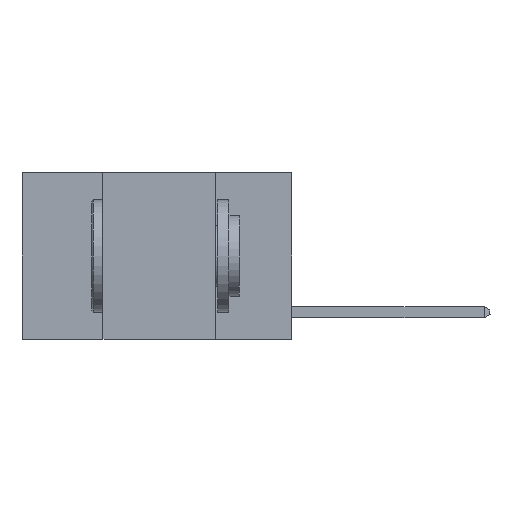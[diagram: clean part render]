
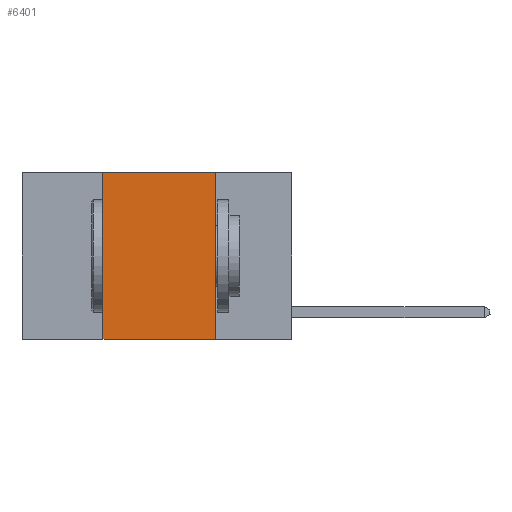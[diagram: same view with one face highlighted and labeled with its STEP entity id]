
A CAD part, left-side view. The second image highlights one B-rep face of the part: STEP entity #6401.
In plain terms, the highlighted planar face has unit normal (-1, 0, 0).
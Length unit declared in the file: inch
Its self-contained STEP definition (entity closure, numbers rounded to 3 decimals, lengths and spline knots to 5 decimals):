
#326 = CARTESIAN_POINT ( 'NONE',  ( 0., 0.42, 0. ) ) ;
#2627 = VECTOR ( 'NONE', #6405, 39.37008 ) ;
#2744 = CARTESIAN_POINT ( 'NONE',  ( 0., 0.17, -0.37 ) ) ;
#3440 = VERTEX_POINT ( 'NONE', #12475 ) ;
#3453 = VERTEX_POINT ( 'NONE', #2744 ) ;
#3882 = LINE ( 'NONE', #13676, #13071 ) ;
#4671 = ORIENTED_EDGE ( 'NONE', *, *, #11369, .T. ) ;
#5184 = CARTESIAN_POINT ( 'NONE',  ( 0., 0.6, 0. ) ) ;
#5519 = CARTESIAN_POINT ( 'NONE',  ( 0., 0.6, 0. ) ) ;
#5595 = EDGE_LOOP ( 'NONE', ( #15292, #9156, #9131, #4671 ) ) ;
#5746 = DIRECTION ( 'NONE',  ( 0., -1., 0. ) ) ;
#6401 = ADVANCED_FACE ( 'NONE', ( #8897 ), #11085, .F. ) ;
#6405 = DIRECTION ( 'NONE',  ( 0., 0., 1. ) ) ;
#6480 = LINE ( 'NONE', #12525, #2627 ) ;
#6493 = DIRECTION ( 'NONE',  ( 0., 0., -1. ) ) ;
#6754 = LINE ( 'NONE', #5519, #8022 ) ;
#7380 = CARTESIAN_POINT ( 'NONE',  ( 0., 0.17, 0. ) ) ;
#8022 = VECTOR ( 'NONE', #5746, 39.37008 ) ;
#8108 = EDGE_CURVE ( 'NONE', #14585, #9340, #6480, .T. ) ;
#8481 = DIRECTION ( 'NONE',  ( 0., 0., -1. ) ) ;
#8618 = DIRECTION ( 'NONE',  ( 0., -1., 0. ) ) ;
#8897 = FACE_OUTER_BOUND ( 'NONE', #5595, .T. ) ;
#9016 = CARTESIAN_POINT ( 'NONE',  ( 0., 0.42, -0.37 ) ) ;
#9131 = ORIENTED_EDGE ( 'NONE', *, *, #8108, .F. ) ;
#9156 = ORIENTED_EDGE ( 'NONE', *, *, #12716, .F. ) ;
#9340 = VERTEX_POINT ( 'NONE', #326 ) ;
#9930 = DIRECTION ( 'NONE',  ( 1., 0., 0. ) ) ;
#11085 = PLANE ( 'NONE',  #12470 ) ;
#11369 = EDGE_CURVE ( 'NONE', #14585, #3453, #3882, .T. ) ;
#12269 = LINE ( 'NONE', #7380, #13871 ) ;
#12397 = EDGE_CURVE ( 'NONE', #3440, #3453, #12269, .T. ) ;
#12470 = AXIS2_PLACEMENT_3D ( 'NONE', #5184, #9930, #6493 ) ;
#12475 = CARTESIAN_POINT ( 'NONE',  ( 0., 0.17, 0. ) ) ;
#12525 = CARTESIAN_POINT ( 'NONE',  ( 0., 0.42, 0. ) ) ;
#12716 = EDGE_CURVE ( 'NONE', #9340, #3440, #6754, .T. ) ;
#13071 = VECTOR ( 'NONE', #8618, 39.37008 ) ;
#13676 = CARTESIAN_POINT ( 'NONE',  ( 0., 0.6, -0.37 ) ) ;
#13871 = VECTOR ( 'NONE', #8481, 39.37008 ) ;
#14585 = VERTEX_POINT ( 'NONE', #9016 ) ;
#15292 = ORIENTED_EDGE ( 'NONE', *, *, #12397, .F. ) ;
